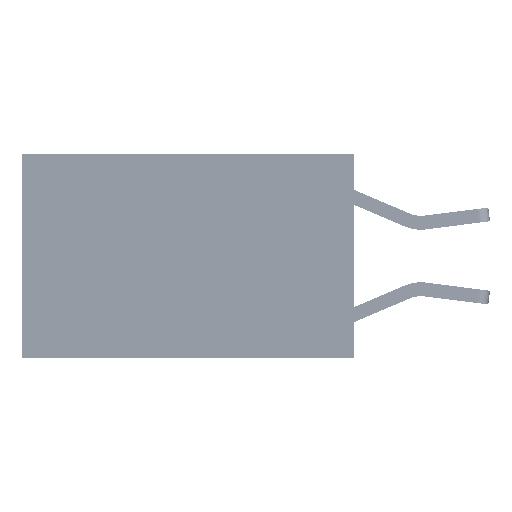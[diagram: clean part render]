
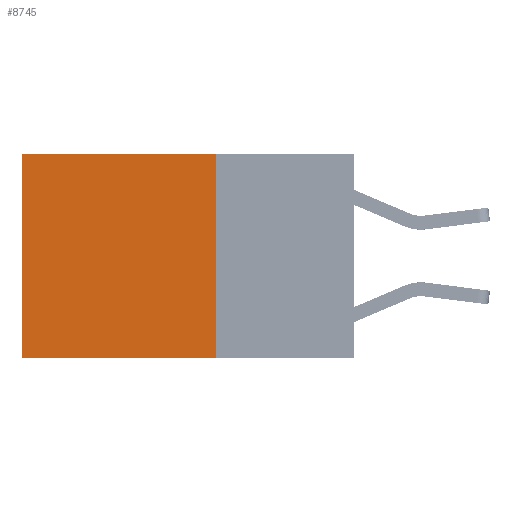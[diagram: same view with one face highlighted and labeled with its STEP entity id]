
A CAD part, left-side view. The second image highlights one B-rep face of the part: STEP entity #8745.
In plain terms, the highlighted planar face has unit normal (-1, 0, 0).
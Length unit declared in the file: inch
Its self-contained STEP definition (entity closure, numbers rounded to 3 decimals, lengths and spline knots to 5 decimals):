
#999 = DIRECTION ( 'NONE',  ( 0., 0., -1. ) ) ;
#1095 = LINE ( 'NONE', #3484, #26814 ) ;
#1771 = ORIENTED_EDGE ( 'NONE', *, *, #8679, .F. ) ;
#1915 = ORIENTED_EDGE ( 'NONE', *, *, #24277, .T. ) ;
#2020 = EDGE_CURVE ( 'NONE', #8126, #11116, #8766, .T. ) ;
#2097 = VECTOR ( 'NONE', #23176, 39.37008 ) ;
#3484 = CARTESIAN_POINT ( 'NONE',  ( 0.2625, 0.25, -0.37 ) ) ;
#4397 = CARTESIAN_POINT ( 'NONE',  ( 0.2625, 0.25, 0. ) ) ;
#4878 = LINE ( 'NONE', #7552, #7510 ) ;
#6149 = CARTESIAN_POINT ( 'NONE',  ( 0.2625, 0.25, 0. ) ) ;
#7510 = VECTOR ( 'NONE', #27283, 39.37008 ) ;
#7552 = CARTESIAN_POINT ( 'NONE',  ( 0.2625, 0.25, 0. ) ) ;
#8126 = VERTEX_POINT ( 'NONE', #20396 ) ;
#8679 = EDGE_CURVE ( 'NONE', #28668, #11116, #1095, .T. ) ;
#8707 = PLANE ( 'NONE',  #25801 ) ;
#8745 = ADVANCED_FACE ( 'NONE', ( #22869 ), #8707, .F. ) ;
#8766 = LINE ( 'NONE', #18008, #27499 ) ;
#8789 = ORIENTED_EDGE ( 'NONE', *, *, #2020, .T. ) ;
#9625 = ORIENTED_EDGE ( 'NONE', *, *, #21140, .F. ) ;
#10797 = DIRECTION ( 'NONE',  ( 0., 0., -1. ) ) ;
#11116 = VERTEX_POINT ( 'NONE', #23599 ) ;
#13400 = CARTESIAN_POINT ( 'NONE',  ( 0.2625, 0.25, -0.37 ) ) ;
#15887 = DIRECTION ( 'NONE',  ( 1., 0., 0. ) ) ;
#18008 = CARTESIAN_POINT ( 'NONE',  ( 0.2625, 0.6, 0. ) ) ;
#20396 = CARTESIAN_POINT ( 'NONE',  ( 0.2625, 0.6, 0. ) ) ;
#21111 = VERTEX_POINT ( 'NONE', #29349 ) ;
#21140 = EDGE_CURVE ( 'NONE', #21111, #28668, #4878, .T. ) ;
#22869 = FACE_OUTER_BOUND ( 'NONE', #27849, .T. ) ;
#23176 = DIRECTION ( 'NONE',  ( 0., 1., 0. ) ) ;
#23599 = CARTESIAN_POINT ( 'NONE',  ( 0.2625, 0.6, -0.37 ) ) ;
#24277 = EDGE_CURVE ( 'NONE', #21111, #8126, #26185, .T. ) ;
#25801 = AXIS2_PLACEMENT_3D ( 'NONE', #6149, #15887, #10797 ) ;
#26185 = LINE ( 'NONE', #4397, #2097 ) ;
#26814 = VECTOR ( 'NONE', #30494, 39.37008 ) ;
#27283 = DIRECTION ( 'NONE',  ( 0., 0., -1. ) ) ;
#27499 = VECTOR ( 'NONE', #999, 39.37008 ) ;
#27849 = EDGE_LOOP ( 'NONE', ( #8789, #1771, #9625, #1915 ) ) ;
#28668 = VERTEX_POINT ( 'NONE', #13400 ) ;
#29349 = CARTESIAN_POINT ( 'NONE',  ( 0.2625, 0.25, 0. ) ) ;
#30494 = DIRECTION ( 'NONE',  ( 0., 1., 0. ) ) ;
